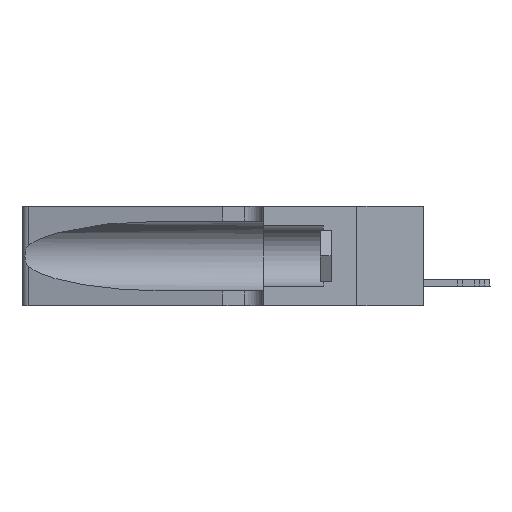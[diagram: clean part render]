
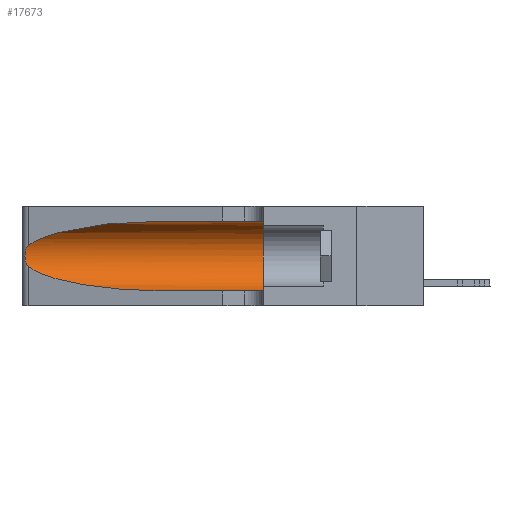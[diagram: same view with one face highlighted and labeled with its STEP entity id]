
A CAD part, left-side view. The second image highlights one B-rep face of the part: STEP entity #17673.
In plain terms, the highlighted cylindrical face has radius 3.308 mm (diameter 6.617 mm), a partial arc.
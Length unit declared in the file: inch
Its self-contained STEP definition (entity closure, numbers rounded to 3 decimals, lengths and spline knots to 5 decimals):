
#336 = VERTEX_POINT ( 'NONE', #45133 ) ;
#1670 = CARTESIAN_POINT ( 'NONE',  ( 0.1305, 0.35, 0.185 ) ) ;
#2416 = CARTESIAN_POINT ( 'NONE',  ( 0.25487, 1.22718, 0.22369 ) ) ;
#5949 = CARTESIAN_POINT ( 'NONE',  ( 0.1305, 0.72297, 0.31525 ) ) ;
#6598 = CARTESIAN_POINT ( 'NONE',  ( 0.25639, 1.23184, 0.21858 ) ) ;
#6774 = LINE ( 'NONE', #31116, #48718 ) ;
#7814 = CYLINDRICAL_SURFACE ( 'NONE', #38481, 0.13025 ) ;
#8262 = CARTESIAN_POINT ( 'NONE',  ( 0.25487, 1.22718, 0.22369 ) ) ;
#8640 = EDGE_LOOP ( 'NONE', ( #42479, #37114, #49740, #10618, #15951, #44477 ) ) ;
#8976 = VERTEX_POINT ( 'NONE', #45908 ) ;
#9004 = CARTESIAN_POINT ( 'NONE',  ( 0.2373, 1.15595, 0.08982 ) ) ;
#10273 = CARTESIAN_POINT ( 'NONE',  ( 0.26075, 1.23896, 0.178 ) ) ;
#10618 = ORIENTED_EDGE ( 'NONE', *, *, #15657, .T. ) ;
#11072 = EDGE_CURVE ( 'NONE', #26227, #8976, #50274, .T. ) ;
#12933 = CARTESIAN_POINT ( 'NONE',  ( 0.25854, 1.2359, 0.20912 ) ) ;
#14015 =( BOUNDED_CURVE ( )  B_SPLINE_CURVE ( 3, ( #47455, #9004, #24674, #36413 ),
 .UNSPECIFIED., .F., .T. ) 
 B_SPLINE_CURVE_WITH_KNOTS ( ( 4, 4 ),
 ( 3.44316, 4.71239 ),
 .UNSPECIFIED. ) 
 CURVE ( )  GEOMETRIC_REPRESENTATION_ITEM ( )  RATIONAL_B_SPLINE_CURVE ( ( 1., 0.87, 0.87, 1. ) ) 
 REPRESENTATION_ITEM ( '' )  );
#14971 = B_SPLINE_CURVE_WITH_KNOTS ( 'NONE', 3,
 ( #36623, #32051, #6598, #19782, #12933, #24145, #32185, #10273, #32257, #35372, #22405, #16626, #31997, #28757 ),
 .UNSPECIFIED., .F., .F.,
 ( 4, 2, 2, 2, 2, 2, 4 ),
 ( 0., 0.00027, 0.00053, 0.00107, 0.0016, 0.00187, 0.00214 ),
 .UNSPECIFIED. ) ;
#15657 = EDGE_CURVE ( 'NONE', #32063, #8976, #39954, .T. ) ;
#15951 = ORIENTED_EDGE ( 'NONE', *, *, #11072, .F. ) ;
#16626 = CARTESIAN_POINT ( 'NONE',  ( 0.25639, 1.23186, 0.15144 ) ) ;
#16932 = CARTESIAN_POINT ( 'NONE',  ( 0.1305, 0.72297, 0.05475 ) ) ;
#17673 = ADVANCED_FACE ( 'NONE', ( #18787 ), #7814, .F. ) ;
#17922 = DIRECTION ( 'NONE',  ( 0., 1., 0. ) ) ;
#18787 = FACE_OUTER_BOUND ( 'NONE', #8640, .T. ) ;
#19782 = CARTESIAN_POINT ( 'NONE',  ( 0.25787, 1.23484, 0.2124 ) ) ;
#22405 = CARTESIAN_POINT ( 'NONE',  ( 0.25789, 1.23486, 0.15765 ) ) ;
#23933 = VERTEX_POINT ( 'NONE', #2416 ) ;
#24145 = CARTESIAN_POINT ( 'NONE',  ( 0.26018, 1.23835, 0.19895 ) ) ;
#24335 = VERTEX_POINT ( 'NONE', #5949 ) ;
#24674 = CARTESIAN_POINT ( 'NONE',  ( 0.18966, 0.96281, 0.05475 ) ) ;
#26227 = VERTEX_POINT ( 'NONE', #47569 ) ;
#26733 = CARTESIAN_POINT ( 'NONE',  ( 0.1305, 1.61858, 0.05475 ) ) ;
#27512 = CARTESIAN_POINT ( 'NONE',  ( 0.1305, 0.72297, 0.31525 ) ) ;
#28274 = EDGE_CURVE ( 'NONE', #336, #32063, #14015, .T. ) ;
#28757 = CARTESIAN_POINT ( 'NONE',  ( 0.25487, 1.22718, 0.14631 ) ) ;
#29629 = EDGE_CURVE ( 'NONE', #23933, #336, #14971, .T. ) ;
#30864 =( BOUNDED_CURVE ( )  B_SPLINE_CURVE ( 3, ( #27512, #31597, #47498, #8262 ),
 .UNSPECIFIED., .F., .T. ) 
 B_SPLINE_CURVE_WITH_KNOTS ( ( 4, 4 ),
 ( 1.5708, 2.84003 ),
 .UNSPECIFIED. ) 
 CURVE ( )  GEOMETRIC_REPRESENTATION_ITEM ( )  RATIONAL_B_SPLINE_CURVE ( ( 1., 0.87, 0.87, 1. ) ) 
 REPRESENTATION_ITEM ( '' )  );
#31116 = CARTESIAN_POINT ( 'NONE',  ( 0.1305, 1.61858, 0.31525 ) ) ;
#31597 = CARTESIAN_POINT ( 'NONE',  ( 0.18966, 0.96281, 0.31525 ) ) ;
#31997 = CARTESIAN_POINT ( 'NONE',  ( 0.25555, 1.22993, 0.14849 ) ) ;
#32051 = CARTESIAN_POINT ( 'NONE',  ( 0.25555, 1.22994, 0.2215 ) ) ;
#32063 = VERTEX_POINT ( 'NONE', #16932 ) ;
#32185 = CARTESIAN_POINT ( 'NONE',  ( 0.26075, 1.23896, 0.19203 ) ) ;
#32257 = CARTESIAN_POINT ( 'NONE',  ( 0.26017, 1.23833, 0.17102 ) ) ;
#33047 = DIRECTION ( 'NONE',  ( 0., 0., 1. ) ) ;
#34719 = DIRECTION ( 'NONE',  ( 0., -1., 0. ) ) ;
#35372 = CARTESIAN_POINT ( 'NONE',  ( 0.25856, 1.23593, 0.16098 ) ) ;
#36413 = CARTESIAN_POINT ( 'NONE',  ( 0.1305, 0.72297, 0.05475 ) ) ;
#36567 = CARTESIAN_POINT ( 'NONE',  ( 0.1305, 1.61858, 0.185 ) ) ;
#36623 = CARTESIAN_POINT ( 'NONE',  ( 0.25487, 1.22718, 0.22369 ) ) ;
#37114 = ORIENTED_EDGE ( 'NONE', *, *, #29629, .T. ) ;
#38481 = AXIS2_PLACEMENT_3D ( 'NONE', #36567, #48268, #44005 ) ;
#39343 = VECTOR ( 'NONE', #34719, 39.37008 ) ;
#39954 = LINE ( 'NONE', #26733, #39343 ) ;
#41152 = EDGE_CURVE ( 'NONE', #24335, #26227, #6774, .T. ) ;
#42479 = ORIENTED_EDGE ( 'NONE', *, *, #46195, .T. ) ;
#43236 = AXIS2_PLACEMENT_3D ( 'NONE', #1670, #17922, #33047 ) ;
#44005 = DIRECTION ( 'NONE',  ( 0., 0., -1. ) ) ;
#44477 = ORIENTED_EDGE ( 'NONE', *, *, #41152, .F. ) ;
#44805 = DIRECTION ( 'NONE',  ( 0., -1., 0. ) ) ;
#45133 = CARTESIAN_POINT ( 'NONE',  ( 0.25487, 1.22718, 0.14631 ) ) ;
#45908 = CARTESIAN_POINT ( 'NONE',  ( 0.1305, 0.35, 0.05475 ) ) ;
#46195 = EDGE_CURVE ( 'NONE', #24335, #23933, #30864, .T. ) ;
#47455 = CARTESIAN_POINT ( 'NONE',  ( 0.25487, 1.22718, 0.14631 ) ) ;
#47498 = CARTESIAN_POINT ( 'NONE',  ( 0.2373, 1.15595, 0.28018 ) ) ;
#47569 = CARTESIAN_POINT ( 'NONE',  ( 0.1305, 0.35, 0.31525 ) ) ;
#48268 = DIRECTION ( 'NONE',  ( 0., -1., 0. ) ) ;
#48718 = VECTOR ( 'NONE', #44805, 39.37008 ) ;
#49740 = ORIENTED_EDGE ( 'NONE', *, *, #28274, .T. ) ;
#50274 = CIRCLE ( 'NONE', #43236, 0.13025 ) ;
